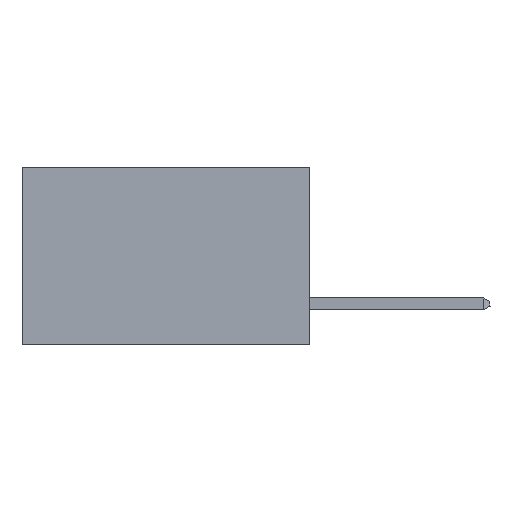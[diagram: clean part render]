
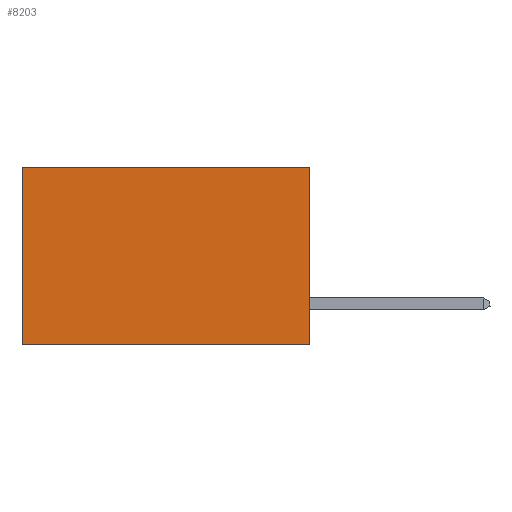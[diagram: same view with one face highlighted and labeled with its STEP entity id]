
A CAD part, left-side view. The second image highlights one B-rep face of the part: STEP entity #8203.
In plain terms, the highlighted planar face has unit normal (-1, 0, 0).
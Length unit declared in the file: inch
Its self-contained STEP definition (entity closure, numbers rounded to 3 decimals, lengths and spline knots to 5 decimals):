
#2922 = VECTOR ( 'NONE', #6329, 39.37008 ) ;
#6329 = DIRECTION ( 'NONE',  ( 0., 0., -1. ) ) ;
#7666 = CARTESIAN_POINT ( 'NONE',  ( 0.2875, 0.6, 0. ) ) ;
#8203 = ADVANCED_FACE ( 'NONE', ( #24049 ), #32054, .F. ) ;
#11661 = CARTESIAN_POINT ( 'NONE',  ( 0.2875, 0., -0.37 ) ) ;
#15012 = DIRECTION ( 'NONE',  ( 0., 1., 0. ) ) ;
#15577 = ORIENTED_EDGE ( 'NONE', *, *, #31431, .F. ) ;
#15661 = DIRECTION ( 'NONE',  ( 0., 1., 0. ) ) ;
#15724 = LINE ( 'NONE', #26796, #30853 ) ;
#17941 = VECTOR ( 'NONE', #15661, 39.37008 ) ;
#18031 = VECTOR ( 'NONE', #15012, 39.37008 ) ;
#18899 = EDGE_CURVE ( 'NONE', #36749, #37851, #33117, .T. ) ;
#18967 = LINE ( 'NONE', #28238, #17941 ) ;
#19093 = ORIENTED_EDGE ( 'NONE', *, *, #18899, .F. ) ;
#19346 = EDGE_LOOP ( 'NONE', ( #36004, #19093, #15577, #37822 ) ) ;
#19497 = CARTESIAN_POINT ( 'NONE',  ( 0.2875, 0.6, 0. ) ) ;
#19889 = CARTESIAN_POINT ( 'NONE',  ( 0.2875, 0., 0. ) ) ;
#20229 = DIRECTION ( 'NONE',  ( 0., 0., -1. ) ) ;
#22798 = AXIS2_PLACEMENT_3D ( 'NONE', #38822, #39574, #20229 ) ;
#23942 = EDGE_CURVE ( 'NONE', #27949, #37851, #34821, .T. ) ;
#24049 = FACE_OUTER_BOUND ( 'NONE', #19346, .T. ) ;
#24192 = CARTESIAN_POINT ( 'NONE',  ( 0.2875, 0.6, -0.37 ) ) ;
#24840 = CARTESIAN_POINT ( 'NONE',  ( 0.2875, 0., -0.37 ) ) ;
#26330 = EDGE_CURVE ( 'NONE', #35910, #27949, #18967, .T. ) ;
#26796 = CARTESIAN_POINT ( 'NONE',  ( 0.2875, 0., 0. ) ) ;
#27949 = VERTEX_POINT ( 'NONE', #7666 ) ;
#28238 = CARTESIAN_POINT ( 'NONE',  ( 0.2875, 0., 0. ) ) ;
#30853 = VECTOR ( 'NONE', #36718, 39.37008 ) ;
#31431 = EDGE_CURVE ( 'NONE', #35910, #36749, #15724, .T. ) ;
#32054 = PLANE ( 'NONE',  #22798 ) ;
#33117 = LINE ( 'NONE', #11661, #18031 ) ;
#34821 = LINE ( 'NONE', #19497, #2922 ) ;
#35910 = VERTEX_POINT ( 'NONE', #19889 ) ;
#36004 = ORIENTED_EDGE ( 'NONE', *, *, #23942, .T. ) ;
#36718 = DIRECTION ( 'NONE',  ( 0., 0., -1. ) ) ;
#36749 = VERTEX_POINT ( 'NONE', #24840 ) ;
#37822 = ORIENTED_EDGE ( 'NONE', *, *, #26330, .T. ) ;
#37851 = VERTEX_POINT ( 'NONE', #24192 ) ;
#38822 = CARTESIAN_POINT ( 'NONE',  ( 0.2875, 0., 0. ) ) ;
#39574 = DIRECTION ( 'NONE',  ( 1., 0., 0. ) ) ;
